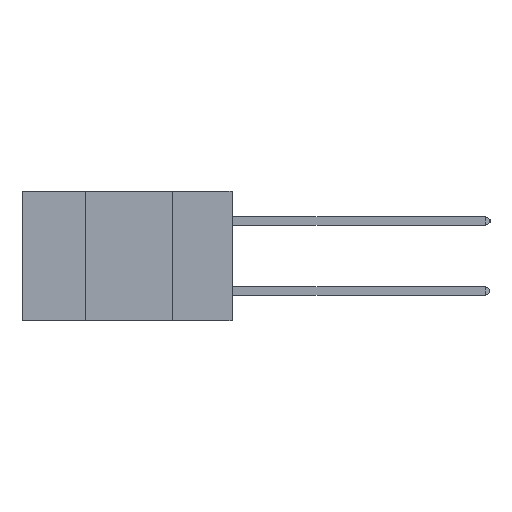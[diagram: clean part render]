
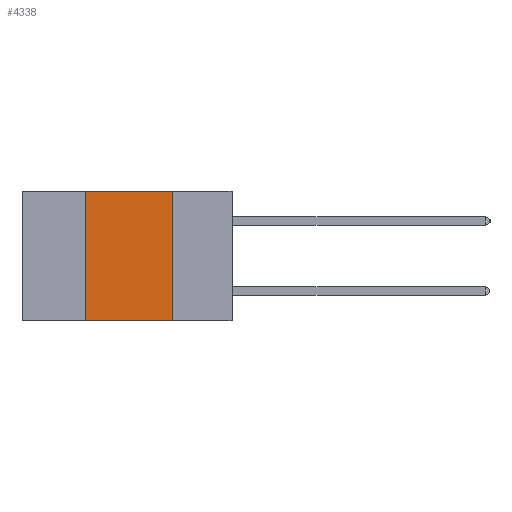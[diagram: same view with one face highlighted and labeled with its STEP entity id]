
A CAD part, left-side view. The second image highlights one B-rep face of the part: STEP entity #4338.
In plain terms, the highlighted planar face has unit normal (-1, 0, 0).
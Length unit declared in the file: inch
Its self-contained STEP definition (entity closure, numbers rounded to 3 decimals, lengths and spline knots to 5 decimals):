
#56 = EDGE_CURVE ( 'NONE', #16085, #4641, #7183, .T. ) ;
#978 = CARTESIAN_POINT ( 'NONE',  ( 0., 0.17, -0.37 ) ) ;
#1660 = ORIENTED_EDGE ( 'NONE', *, *, #56, .F. ) ;
#2394 = CARTESIAN_POINT ( 'NONE',  ( 0., 0.17, 0. ) ) ;
#3281 = VERTEX_POINT ( 'NONE', #20763 ) ;
#4338 = ADVANCED_FACE ( 'NONE', ( #20209 ), #19171, .F. ) ;
#4641 = VERTEX_POINT ( 'NONE', #2394 ) ;
#4956 = ORIENTED_EDGE ( 'NONE', *, *, #18041, .F. ) ;
#5106 = CARTESIAN_POINT ( 'NONE',  ( 0., 0.6, -0.37 ) ) ;
#5228 = DIRECTION ( 'NONE',  ( 0., -1., 0. ) ) ;
#5368 = EDGE_CURVE ( 'NONE', #3281, #15213, #9186, .T. ) ;
#5873 = CARTESIAN_POINT ( 'NONE',  ( 0., 0.42, 0. ) ) ;
#6115 = VECTOR ( 'NONE', #15086, 39.37008 ) ;
#6762 = DIRECTION ( 'NONE',  ( 0., 0., -1. ) ) ;
#7183 = LINE ( 'NONE', #10955, #6115 ) ;
#7509 = ORIENTED_EDGE ( 'NONE', *, *, #10486, .F. ) ;
#7538 = ORIENTED_EDGE ( 'NONE', *, *, #5368, .T. ) ;
#8619 = CARTESIAN_POINT ( 'NONE',  ( 0., 0.42, 0. ) ) ;
#9186 = LINE ( 'NONE', #5106, #21413 ) ;
#9215 = DIRECTION ( 'NONE',  ( 0., 0., 1. ) ) ;
#10486 = EDGE_CURVE ( 'NONE', #3281, #16085, #19962, .T. ) ;
#10955 = CARTESIAN_POINT ( 'NONE',  ( 0., 0.6, 0. ) ) ;
#11057 = EDGE_LOOP ( 'NONE', ( #4956, #1660, #7509, #7538 ) ) ;
#13299 = LINE ( 'NONE', #16415, #17582 ) ;
#15086 = DIRECTION ( 'NONE',  ( 0., -1., 0. ) ) ;
#15213 = VERTEX_POINT ( 'NONE', #978 ) ;
#15740 = VECTOR ( 'NONE', #9215, 39.37008 ) ;
#16085 = VERTEX_POINT ( 'NONE', #8619 ) ;
#16415 = CARTESIAN_POINT ( 'NONE',  ( 0., 0.17, 0. ) ) ;
#17582 = VECTOR ( 'NONE', #6762, 39.37008 ) ;
#18041 = EDGE_CURVE ( 'NONE', #4641, #15213, #13299, .T. ) ;
#18322 = AXIS2_PLACEMENT_3D ( 'NONE', #20117, #19153, #18901 ) ;
#18901 = DIRECTION ( 'NONE',  ( 0., 0., -1. ) ) ;
#19153 = DIRECTION ( 'NONE',  ( 1., 0., 0. ) ) ;
#19171 = PLANE ( 'NONE',  #18322 ) ;
#19962 = LINE ( 'NONE', #5873, #15740 ) ;
#20117 = CARTESIAN_POINT ( 'NONE',  ( 0., 0.6, 0. ) ) ;
#20209 = FACE_OUTER_BOUND ( 'NONE', #11057, .T. ) ;
#20763 = CARTESIAN_POINT ( 'NONE',  ( 0., 0.42, -0.37 ) ) ;
#21413 = VECTOR ( 'NONE', #5228, 39.37008 ) ;
